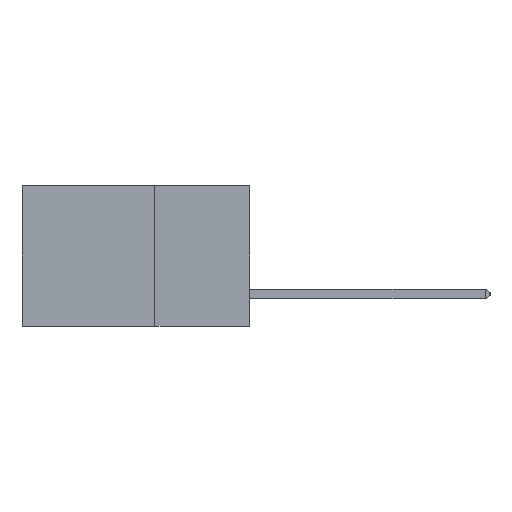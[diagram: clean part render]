
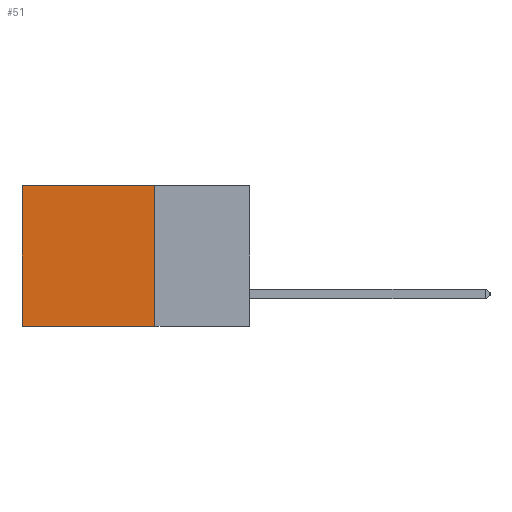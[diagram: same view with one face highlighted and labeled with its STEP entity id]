
A CAD part, left-side view. The second image highlights one B-rep face of the part: STEP entity #51.
In plain terms, the highlighted planar face has unit normal (-1, 0, 0).
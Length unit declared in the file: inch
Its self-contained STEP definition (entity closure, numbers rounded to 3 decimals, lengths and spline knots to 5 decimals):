
#51 = ADVANCED_FACE ( 'NONE', ( #19477 ), #2156, .F. ) ;
#1063 = VECTOR ( 'NONE', #2648, 39.37008 ) ;
#1279 = VERTEX_POINT ( 'NONE', #15407 ) ;
#2156 = PLANE ( 'NONE',  #13882 ) ;
#2177 = CARTESIAN_POINT ( 'NONE',  ( 0.2875, 0.25, 0. ) ) ;
#2246 = VECTOR ( 'NONE', #17430, 39.37008 ) ;
#2378 = DIRECTION ( 'NONE',  ( 0., 0., -1. ) ) ;
#2443 = DIRECTION ( 'NONE',  ( 1., 0., 0. ) ) ;
#2648 = DIRECTION ( 'NONE',  ( 0., 1., 0. ) ) ;
#2709 = EDGE_CURVE ( 'NONE', #3848, #11332, #5366, .T. ) ;
#3023 = CARTESIAN_POINT ( 'NONE',  ( 0.2875, 0.25, 0. ) ) ;
#3103 = EDGE_CURVE ( 'NONE', #3848, #9858, #6858, .T. ) ;
#3848 = VERTEX_POINT ( 'NONE', #7212 ) ;
#5366 = LINE ( 'NONE', #3023, #1063 ) ;
#6016 = CARTESIAN_POINT ( 'NONE',  ( 0.2875, 0.6, 0. ) ) ;
#6397 = LINE ( 'NONE', #17135, #14309 ) ;
#6443 = CARTESIAN_POINT ( 'NONE',  ( 0.2875, 0.25, -0.37 ) ) ;
#6520 = LINE ( 'NONE', #6443, #2246 ) ;
#6858 = LINE ( 'NONE', #15538, #14759 ) ;
#7212 = CARTESIAN_POINT ( 'NONE',  ( 0.2875, 0.25, 0. ) ) ;
#7850 = CARTESIAN_POINT ( 'NONE',  ( 0.2875, 0.25, -0.37 ) ) ;
#8327 = ORIENTED_EDGE ( 'NONE', *, *, #2709, .T. ) ;
#8771 = EDGE_CURVE ( 'NONE', #9858, #1279, #6520, .T. ) ;
#9314 = DIRECTION ( 'NONE',  ( 0., 0., -1. ) ) ;
#9858 = VERTEX_POINT ( 'NONE', #7850 ) ;
#11332 = VERTEX_POINT ( 'NONE', #6016 ) ;
#12041 = EDGE_CURVE ( 'NONE', #11332, #1279, #6397, .T. ) ;
#13021 = DIRECTION ( 'NONE',  ( 0., 0., -1. ) ) ;
#13211 = ORIENTED_EDGE ( 'NONE', *, *, #3103, .F. ) ;
#13882 = AXIS2_PLACEMENT_3D ( 'NONE', #2177, #2443, #2378 ) ;
#14309 = VECTOR ( 'NONE', #9314, 39.37008 ) ;
#14759 = VECTOR ( 'NONE', #13021, 39.37008 ) ;
#15407 = CARTESIAN_POINT ( 'NONE',  ( 0.2875, 0.6, -0.37 ) ) ;
#15538 = CARTESIAN_POINT ( 'NONE',  ( 0.2875, 0.25, 0. ) ) ;
#15768 = EDGE_LOOP ( 'NONE', ( #18548, #18552, #13211, #8327 ) ) ;
#17135 = CARTESIAN_POINT ( 'NONE',  ( 0.2875, 0.6, 0. ) ) ;
#17430 = DIRECTION ( 'NONE',  ( 0., 1., 0. ) ) ;
#18548 = ORIENTED_EDGE ( 'NONE', *, *, #12041, .T. ) ;
#18552 = ORIENTED_EDGE ( 'NONE', *, *, #8771, .F. ) ;
#19477 = FACE_OUTER_BOUND ( 'NONE', #15768, .T. ) ;
